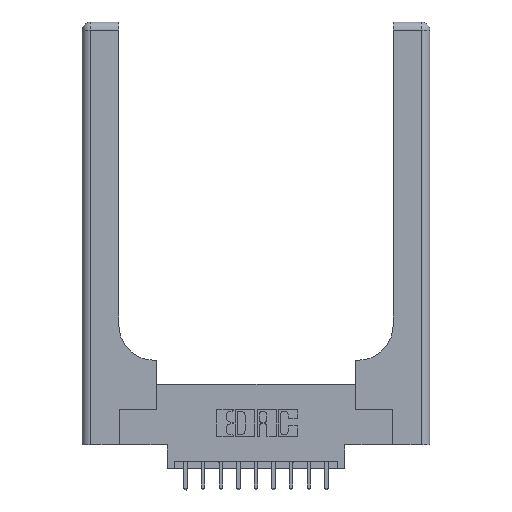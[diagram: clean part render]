
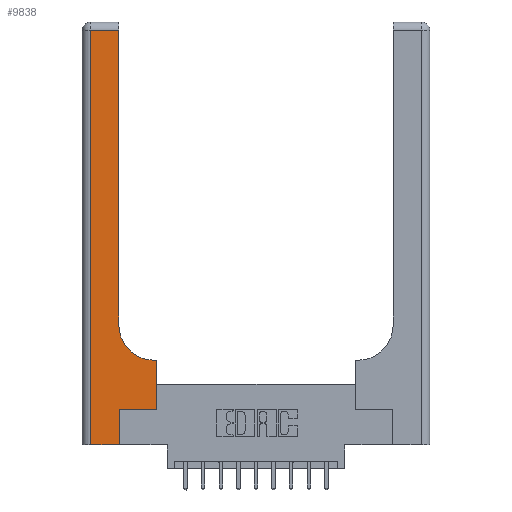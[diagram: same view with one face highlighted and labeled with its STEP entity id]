
A CAD part, top view. The second image highlights one B-rep face of the part: STEP entity #9838.
In plain terms, the highlighted planar face has unit normal (0, 0, 1).
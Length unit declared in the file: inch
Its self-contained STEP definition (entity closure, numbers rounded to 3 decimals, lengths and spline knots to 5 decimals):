
#30 = DIRECTION ( 'NONE',  ( -1., 0., 0. ) ) ;
#79 = VECTOR ( 'NONE', #11075, 39.37008 ) ;
#199 = CARTESIAN_POINT ( 'NONE',  ( 0.528, 0.25, 0.37 ) ) ;
#301 = DIRECTION ( 'NONE',  ( 0., 1., 0. ) ) ;
#461 = VERTEX_POINT ( 'NONE', #8694 ) ;
#745 = LINE ( 'NONE', #10935, #3956 ) ;
#874 = PLANE ( 'NONE',  #2591 ) ;
#1276 = CIRCLE ( 'NONE', #12702, 0.25 ) ;
#1338 = CARTESIAN_POINT ( 'NONE',  ( 0.26, 3., 0.37 ) ) ;
#1459 = ORIENTED_EDGE ( 'NONE', *, *, #10098, .T. ) ;
#1647 = EDGE_CURVE ( 'NONE', #9044, #8799, #745, .T. ) ;
#1843 = VERTEX_POINT ( 'NONE', #12480 ) ;
#2022 = VERTEX_POINT ( 'NONE', #5645 ) ;
#2254 = CARTESIAN_POINT ( 'NONE',  ( 0.06, 0., 0.37 ) ) ;
#2591 = AXIS2_PLACEMENT_3D ( 'NONE', #9314, #10519, #3294 ) ;
#3020 = DIRECTION ( 'NONE',  ( 0., 0., -1. ) ) ;
#3123 = CARTESIAN_POINT ( 'NONE',  ( 0.06, 2.94, 0.37 ) ) ;
#3173 = ORIENTED_EDGE ( 'NONE', *, *, #13583, .T. ) ;
#3283 = LINE ( 'NONE', #4018, #9698 ) ;
#3294 = DIRECTION ( 'NONE',  ( -1., 0., 0. ) ) ;
#3502 = LINE ( 'NONE', #1338, #5934 ) ;
#3690 = CARTESIAN_POINT ( 'NONE',  ( 0.06, 3., 0.37 ) ) ;
#3714 = DIRECTION ( 'NONE',  ( -1., 0., 0. ) ) ;
#3851 = ORIENTED_EDGE ( 'NONE', *, *, #5608, .T. ) ;
#3908 = CARTESIAN_POINT ( 'NONE',  ( 0.26, 2.94, 0.37 ) ) ;
#3956 = VECTOR ( 'NONE', #3714, 39.37008 ) ;
#4018 = CARTESIAN_POINT ( 'NONE',  ( 0., 0., 0.37 ) ) ;
#4263 = VECTOR ( 'NONE', #30, 39.37008 ) ;
#4408 = CARTESIAN_POINT ( 'NONE',  ( 0.265, 0.25, 0.37 ) ) ;
#4450 = LINE ( 'NONE', #3690, #11243 ) ;
#4515 = VECTOR ( 'NONE', #14885, 39.37008 ) ;
#4603 = EDGE_CURVE ( 'NONE', #6968, #7246, #10883, .T. ) ;
#4863 = VECTOR ( 'NONE', #301, 39.37008 ) ;
#5546 = CARTESIAN_POINT ( 'NONE',  ( 0.528, 0.6, 0.37 ) ) ;
#5608 = EDGE_CURVE ( 'NONE', #8799, #13138, #4450, .T. ) ;
#5645 = CARTESIAN_POINT ( 'NONE',  ( 0.51, 0.6, 0.37 ) ) ;
#5713 = EDGE_CURVE ( 'NONE', #14583, #6968, #12950, .T. ) ;
#5934 = VECTOR ( 'NONE', #10992, 39.37008 ) ;
#6493 = FACE_OUTER_BOUND ( 'NONE', #13857, .T. ) ;
#6968 = VERTEX_POINT ( 'NONE', #199 ) ;
#7102 = ORIENTED_EDGE ( 'NONE', *, *, #7742, .T. ) ;
#7246 = VERTEX_POINT ( 'NONE', #5546 ) ;
#7404 = CARTESIAN_POINT ( 'NONE',  ( 0.265, 0.25, 0.37 ) ) ;
#7446 = LINE ( 'NONE', #14519, #4263 ) ;
#7742 = EDGE_CURVE ( 'NONE', #461, #14583, #14157, .T. ) ;
#8694 = CARTESIAN_POINT ( 'NONE',  ( 0.265, 0., 0.37 ) ) ;
#8729 = EDGE_CURVE ( 'NONE', #2022, #1843, #1276, .T. ) ;
#8738 = CARTESIAN_POINT ( 'NONE',  ( 0.528, 0.25, 0.37 ) ) ;
#8799 = VERTEX_POINT ( 'NONE', #3123 ) ;
#9044 = VERTEX_POINT ( 'NONE', #3908 ) ;
#9314 = CARTESIAN_POINT ( 'NONE',  ( 0., 3., 0.37 ) ) ;
#9698 = VECTOR ( 'NONE', #12481, 39.37008 ) ;
#9819 = ORIENTED_EDGE ( 'NONE', *, *, #11527, .T. ) ;
#9838 = ADVANCED_FACE ( 'NONE', ( #6493 ), #874, .F. ) ;
#10047 = CARTESIAN_POINT ( 'NONE',  ( 0.265, 0., 0.37 ) ) ;
#10098 = EDGE_CURVE ( 'NONE', #1843, #9044, #3502, .T. ) ;
#10227 = CARTESIAN_POINT ( 'NONE',  ( 0.51, 0.85, 0.37 ) ) ;
#10519 = DIRECTION ( 'NONE',  ( 0., 0., -1. ) ) ;
#10883 = LINE ( 'NONE', #8738, #4863 ) ;
#10935 = CARTESIAN_POINT ( 'NONE',  ( 0., 2.94, 0.37 ) ) ;
#10992 = DIRECTION ( 'NONE',  ( 0., 1., 0. ) ) ;
#11075 = DIRECTION ( 'NONE',  ( 1., 0., 0. ) ) ;
#11243 = VECTOR ( 'NONE', #12155, 39.37008 ) ;
#11459 = DIRECTION ( 'NONE',  ( 1., 0., 0. ) ) ;
#11527 = EDGE_CURVE ( 'NONE', #13138, #461, #3283, .T. ) ;
#11950 = ORIENTED_EDGE ( 'NONE', *, *, #4603, .T. ) ;
#12155 = DIRECTION ( 'NONE',  ( 0., -1., 0. ) ) ;
#12412 = ORIENTED_EDGE ( 'NONE', *, *, #8729, .T. ) ;
#12480 = CARTESIAN_POINT ( 'NONE',  ( 0.26, 0.85, 0.37 ) ) ;
#12481 = DIRECTION ( 'NONE',  ( 1., 0., 0. ) ) ;
#12552 = ORIENTED_EDGE ( 'NONE', *, *, #1647, .T. ) ;
#12702 = AXIS2_PLACEMENT_3D ( 'NONE', #10227, #3020, #11459 ) ;
#12950 = LINE ( 'NONE', #7404, #79 ) ;
#13138 = VERTEX_POINT ( 'NONE', #2254 ) ;
#13583 = EDGE_CURVE ( 'NONE', #7246, #2022, #7446, .T. ) ;
#13857 = EDGE_LOOP ( 'NONE', ( #1459, #12552, #3851, #9819, #7102, #14814, #11950, #3173, #12412 ) ) ;
#14157 = LINE ( 'NONE', #10047, #4515 ) ;
#14519 = CARTESIAN_POINT ( 'NONE',  ( 0.26, 0.6, 0.37 ) ) ;
#14583 = VERTEX_POINT ( 'NONE', #4408 ) ;
#14814 = ORIENTED_EDGE ( 'NONE', *, *, #5713, .T. ) ;
#14885 = DIRECTION ( 'NONE',  ( 0., 1., 0. ) ) ;
